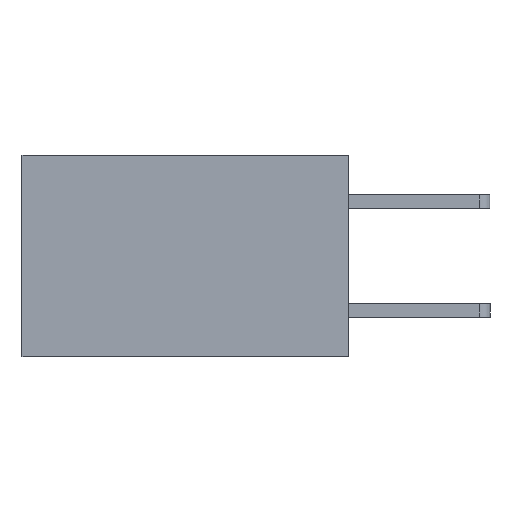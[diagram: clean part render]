
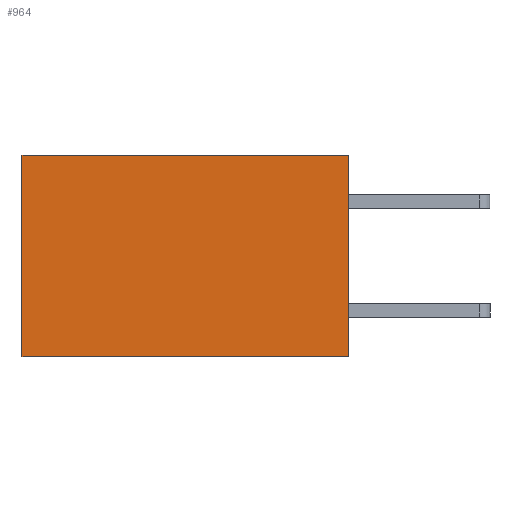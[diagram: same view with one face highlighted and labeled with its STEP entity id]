
A CAD part, left-side view. The second image highlights one B-rep face of the part: STEP entity #964.
In plain terms, the highlighted planar face has unit normal (-1, 0, 0).
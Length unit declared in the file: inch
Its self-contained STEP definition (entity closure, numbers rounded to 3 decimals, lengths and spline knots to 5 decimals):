
#23 = EDGE_CURVE ( 'NONE', #6005, #1128, #96, .T. ) ;
#94 = VECTOR ( 'NONE', #7147, 39.37008 ) ;
#96 = LINE ( 'NONE', #3399, #6644 ) ;
#163 = DIRECTION ( 'NONE',  ( 0., 0., -1. ) ) ;
#301 = ORIENTED_EDGE ( 'NONE', *, *, #23, .T. ) ;
#419 = LINE ( 'NONE', #507, #6933 ) ;
#507 = CARTESIAN_POINT ( 'NONE',  ( 0.2615, 0., -0.37 ) ) ;
#953 = LINE ( 'NONE', #7964, #5655 ) ;
#964 = ADVANCED_FACE ( 'NONE', ( #4731 ), #5069, .F. ) ;
#1128 = VERTEX_POINT ( 'NONE', #6040 ) ;
#1950 = LINE ( 'NONE', #7153, #94 ) ;
#2148 = EDGE_CURVE ( 'NONE', #2897, #3986, #1950, .T. ) ;
#2151 = ORIENTED_EDGE ( 'NONE', *, *, #2357, .T. ) ;
#2291 = DIRECTION ( 'NONE',  ( 0., 1., 0. ) ) ;
#2357 = EDGE_CURVE ( 'NONE', #1128, #3986, #953, .T. ) ;
#2380 = CARTESIAN_POINT ( 'NONE',  ( 0.2615, 0., 0. ) ) ;
#2897 = VERTEX_POINT ( 'NONE', #3572 ) ;
#3363 = EDGE_CURVE ( 'NONE', #6005, #2897, #419, .T. ) ;
#3399 = CARTESIAN_POINT ( 'NONE',  ( 0.2615, 0., 0. ) ) ;
#3572 = CARTESIAN_POINT ( 'NONE',  ( 0.2615, 0., -0.37 ) ) ;
#3714 = ORIENTED_EDGE ( 'NONE', *, *, #2148, .F. ) ;
#3986 = VERTEX_POINT ( 'NONE', #5722 ) ;
#4681 = DIRECTION ( 'NONE',  ( 0., 0., -1. ) ) ;
#4707 = AXIS2_PLACEMENT_3D ( 'NONE', #4969, #4709, #4681 ) ;
#4709 = DIRECTION ( 'NONE',  ( 1., 0., 0. ) ) ;
#4731 = FACE_OUTER_BOUND ( 'NONE', #7754, .T. ) ;
#4969 = CARTESIAN_POINT ( 'NONE',  ( 0.2615, 0., -0.37 ) ) ;
#5069 = PLANE ( 'NONE',  #4707 ) ;
#5655 = VECTOR ( 'NONE', #6660, 39.37008 ) ;
#5722 = CARTESIAN_POINT ( 'NONE',  ( 0.2615, 0.6, -0.37 ) ) ;
#6005 = VERTEX_POINT ( 'NONE', #2380 ) ;
#6040 = CARTESIAN_POINT ( 'NONE',  ( 0.2615, 0.6, 0. ) ) ;
#6644 = VECTOR ( 'NONE', #2291, 39.37008 ) ;
#6660 = DIRECTION ( 'NONE',  ( 0., 0., -1. ) ) ;
#6833 = ORIENTED_EDGE ( 'NONE', *, *, #3363, .F. ) ;
#6933 = VECTOR ( 'NONE', #163, 39.37008 ) ;
#7147 = DIRECTION ( 'NONE',  ( 0., 1., 0. ) ) ;
#7153 = CARTESIAN_POINT ( 'NONE',  ( 0.2615, 0., -0.37 ) ) ;
#7754 = EDGE_LOOP ( 'NONE', ( #2151, #3714, #6833, #301 ) ) ;
#7964 = CARTESIAN_POINT ( 'NONE',  ( 0.2615, 0.6, -0.37 ) ) ;
